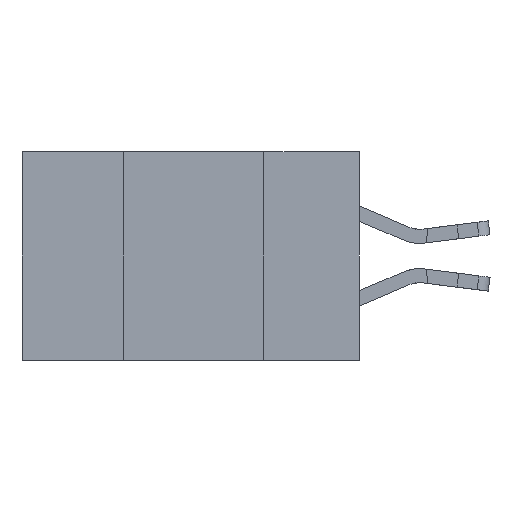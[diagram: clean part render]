
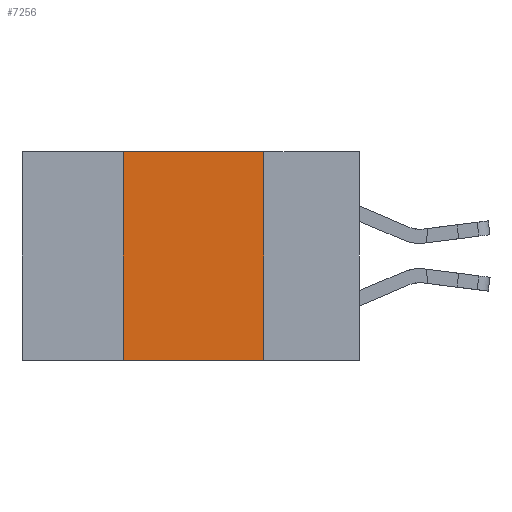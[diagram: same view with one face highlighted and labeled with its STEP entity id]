
A CAD part, left-side view. The second image highlights one B-rep face of the part: STEP entity #7256.
In plain terms, the highlighted planar face has unit normal (-1, 0, 0).
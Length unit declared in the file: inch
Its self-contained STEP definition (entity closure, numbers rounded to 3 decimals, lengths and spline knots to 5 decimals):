
#578 = DIRECTION ( 'NONE',  ( 1., 0., 0. ) ) ;
#642 = ORIENTED_EDGE ( 'NONE', *, *, #2618, .F. ) ;
#1140 = ORIENTED_EDGE ( 'NONE', *, *, #10070, .F. ) ;
#2109 = ORIENTED_EDGE ( 'NONE', *, *, #6476, .T. ) ;
#2260 = VERTEX_POINT ( 'NONE', #2395 ) ;
#2395 = CARTESIAN_POINT ( 'NONE',  ( 0., 0.17, -0.37 ) ) ;
#2618 = EDGE_CURVE ( 'NONE', #10610, #11954, #5048, .T. ) ;
#3394 = CARTESIAN_POINT ( 'NONE',  ( 0., 0.17, 0. ) ) ;
#3712 = CARTESIAN_POINT ( 'NONE',  ( 0., 0.42, 0. ) ) ;
#5048 = LINE ( 'NONE', #23169, #22547 ) ;
#5083 = CARTESIAN_POINT ( 'NONE',  ( 0., 0.17, 0. ) ) ;
#5230 = LINE ( 'NONE', #3712, #23307 ) ;
#5940 = VECTOR ( 'NONE', #21496, 39.37008 ) ;
#6107 = PLANE ( 'NONE',  #8087 ) ;
#6476 = EDGE_CURVE ( 'NONE', #7751, #2260, #21654, .T. ) ;
#6511 = LINE ( 'NONE', #3394, #5940 ) ;
#7256 = ADVANCED_FACE ( 'NONE', ( #14261 ), #6107, .F. ) ;
#7396 = CARTESIAN_POINT ( 'NONE',  ( 0., 0.6, -0.37 ) ) ;
#7669 = EDGE_CURVE ( 'NONE', #7751, #10610, #5230, .T. ) ;
#7751 = VERTEX_POINT ( 'NONE', #9472 ) ;
#7804 = VECTOR ( 'NONE', #19988, 39.37008 ) ;
#8087 = AXIS2_PLACEMENT_3D ( 'NONE', #20518, #578, #13336 ) ;
#9472 = CARTESIAN_POINT ( 'NONE',  ( 0., 0.42, -0.37 ) ) ;
#10070 = EDGE_CURVE ( 'NONE', #11954, #2260, #6511, .T. ) ;
#10610 = VERTEX_POINT ( 'NONE', #12207 ) ;
#11708 = EDGE_LOOP ( 'NONE', ( #1140, #642, #20241, #2109 ) ) ;
#11954 = VERTEX_POINT ( 'NONE', #5083 ) ;
#12207 = CARTESIAN_POINT ( 'NONE',  ( 0., 0.42, 0. ) ) ;
#13336 = DIRECTION ( 'NONE',  ( 0., 0., -1. ) ) ;
#14221 = DIRECTION ( 'NONE',  ( 0., -1., 0. ) ) ;
#14261 = FACE_OUTER_BOUND ( 'NONE', #11708, .T. ) ;
#14524 = DIRECTION ( 'NONE',  ( 0., 0., 1. ) ) ;
#19988 = DIRECTION ( 'NONE',  ( 0., -1., 0. ) ) ;
#20241 = ORIENTED_EDGE ( 'NONE', *, *, #7669, .F. ) ;
#20518 = CARTESIAN_POINT ( 'NONE',  ( 0., 0.6, 0. ) ) ;
#21496 = DIRECTION ( 'NONE',  ( 0., 0., -1. ) ) ;
#21654 = LINE ( 'NONE', #7396, #7804 ) ;
#22547 = VECTOR ( 'NONE', #14221, 39.37008 ) ;
#23169 = CARTESIAN_POINT ( 'NONE',  ( 0., 0.6, 0. ) ) ;
#23307 = VECTOR ( 'NONE', #14524, 39.37008 ) ;
